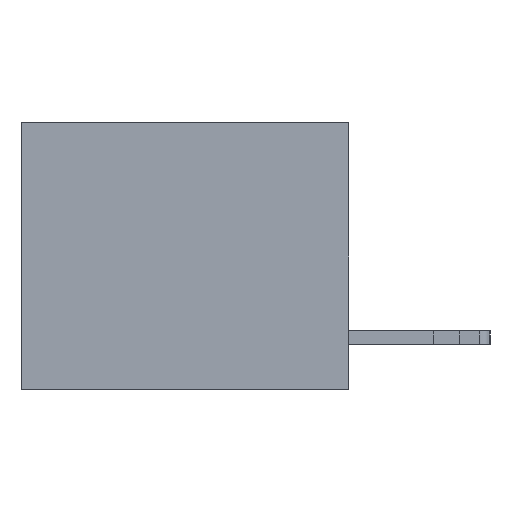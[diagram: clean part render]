
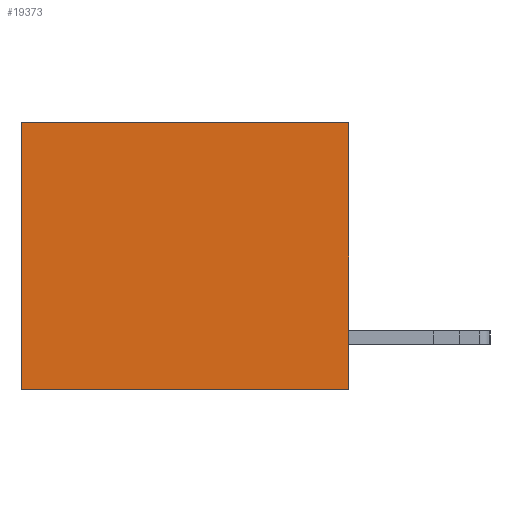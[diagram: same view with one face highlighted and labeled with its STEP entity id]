
A CAD part, left-side view. The second image highlights one B-rep face of the part: STEP entity #19373.
In plain terms, the highlighted planar face has unit normal (-1, 0, 0).
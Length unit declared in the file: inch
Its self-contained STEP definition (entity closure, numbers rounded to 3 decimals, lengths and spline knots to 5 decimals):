
#250 = FACE_OUTER_BOUND ( 'NONE', #10855, .T. ) ;
#281 = VERTEX_POINT ( 'NONE', #4204 ) ;
#751 = VERTEX_POINT ( 'NONE', #9878 ) ;
#825 = CARTESIAN_POINT ( 'NONE',  ( 0.3165, 0., -0.49 ) ) ;
#986 = DIRECTION ( 'NONE',  ( 0., 0., -1. ) ) ;
#1052 = CARTESIAN_POINT ( 'NONE',  ( 0.3165, 0., 0. ) ) ;
#1552 = DIRECTION ( 'NONE',  ( 1., 0., 0. ) ) ;
#1783 = ORIENTED_EDGE ( 'NONE', *, *, #19507, .F. ) ;
#2574 = VECTOR ( 'NONE', #18978, 39.37008 ) ;
#2613 = EDGE_CURVE ( 'NONE', #281, #751, #7027, .T. ) ;
#2625 = ORIENTED_EDGE ( 'NONE', *, *, #2613, .T. ) ;
#4204 = CARTESIAN_POINT ( 'NONE',  ( 0.3165, 0.6, 0. ) ) ;
#5228 = CARTESIAN_POINT ( 'NONE',  ( 0.3165, 0., 0. ) ) ;
#5587 = EDGE_CURVE ( 'NONE', #18220, #281, #20226, .T. ) ;
#5927 = EDGE_CURVE ( 'NONE', #18220, #21522, #22094, .T. ) ;
#7027 = LINE ( 'NONE', #11246, #21984 ) ;
#7799 = CARTESIAN_POINT ( 'NONE',  ( 0.3165, 0., -0.49 ) ) ;
#8090 = ORIENTED_EDGE ( 'NONE', *, *, #5927, .F. ) ;
#9878 = CARTESIAN_POINT ( 'NONE',  ( 0.3165, 0.6, -0.49 ) ) ;
#10051 = DIRECTION ( 'NONE',  ( 0., 0., -1. ) ) ;
#10855 = EDGE_LOOP ( 'NONE', ( #2625, #1783, #8090, #22108 ) ) ;
#11246 = CARTESIAN_POINT ( 'NONE',  ( 0.3165, 0.6, -0.49 ) ) ;
#11853 = DIRECTION ( 'NONE',  ( 0., 0., -1. ) ) ;
#12933 = DIRECTION ( 'NONE',  ( 0., 1., 0. ) ) ;
#13456 = AXIS2_PLACEMENT_3D ( 'NONE', #18709, #1552, #10051 ) ;
#13599 = CARTESIAN_POINT ( 'NONE',  ( 0.3165, 0., -0.49 ) ) ;
#15927 = VECTOR ( 'NONE', #12933, 39.37008 ) ;
#17030 = PLANE ( 'NONE',  #13456 ) ;
#18220 = VERTEX_POINT ( 'NONE', #1052 ) ;
#18709 = CARTESIAN_POINT ( 'NONE',  ( 0.3165, 0., -0.49 ) ) ;
#18803 = VECTOR ( 'NONE', #11853, 39.37008 ) ;
#18978 = DIRECTION ( 'NONE',  ( 0., 1., 0. ) ) ;
#19202 = LINE ( 'NONE', #825, #15927 ) ;
#19373 = ADVANCED_FACE ( 'NONE', ( #250 ), #17030, .F. ) ;
#19507 = EDGE_CURVE ( 'NONE', #21522, #751, #19202, .T. ) ;
#20226 = LINE ( 'NONE', #5228, #2574 ) ;
#21522 = VERTEX_POINT ( 'NONE', #7799 ) ;
#21984 = VECTOR ( 'NONE', #986, 39.37008 ) ;
#22094 = LINE ( 'NONE', #13599, #18803 ) ;
#22108 = ORIENTED_EDGE ( 'NONE', *, *, #5587, .T. ) ;
